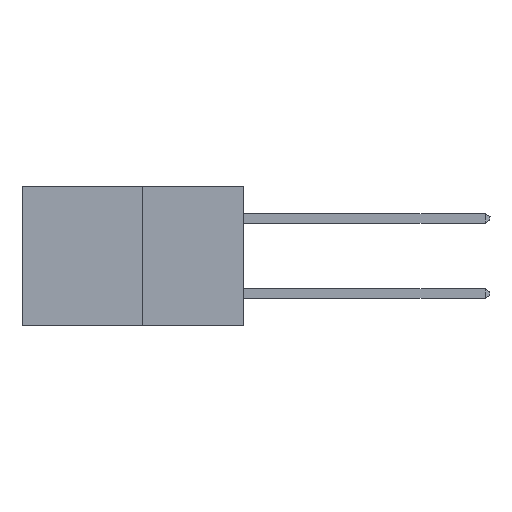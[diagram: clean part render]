
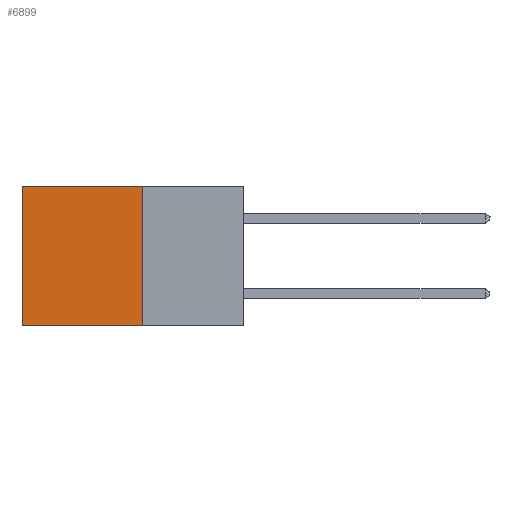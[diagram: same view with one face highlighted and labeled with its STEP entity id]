
A CAD part, left-side view. The second image highlights one B-rep face of the part: STEP entity #6899.
In plain terms, the highlighted planar face has unit normal (-1, 0, 0).
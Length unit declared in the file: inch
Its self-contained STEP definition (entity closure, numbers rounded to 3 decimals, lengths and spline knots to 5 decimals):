
#164 = LINE ( 'NONE', #6016, #4381 ) ;
#496 = VECTOR ( 'NONE', #9819, 39.37008 ) ;
#772 = LINE ( 'NONE', #3320, #496 ) ;
#805 = CARTESIAN_POINT ( 'NONE',  ( 0.277, 0.59, -0.37 ) ) ;
#1192 = DIRECTION ( 'NONE',  ( 0., 1., 0. ) ) ;
#1532 = CARTESIAN_POINT ( 'NONE',  ( 0.277, 0.27, -0.37 ) ) ;
#1769 = ORIENTED_EDGE ( 'NONE', *, *, #7540, .T. ) ;
#2384 = DIRECTION ( 'NONE',  ( 1., 0., 0. ) ) ;
#2575 = ORIENTED_EDGE ( 'NONE', *, *, #4249, .F. ) ;
#2632 = VERTEX_POINT ( 'NONE', #5399 ) ;
#3102 = VECTOR ( 'NONE', #1192, 39.37008 ) ;
#3320 = CARTESIAN_POINT ( 'NONE',  ( 0.277, 0.59, -0.37 ) ) ;
#3494 = EDGE_LOOP ( 'NONE', ( #1769, #8615, #2575, #4795 ) ) ;
#3533 = VERTEX_POINT ( 'NONE', #805 ) ;
#3874 = VERTEX_POINT ( 'NONE', #8811 ) ;
#3890 = LINE ( 'NONE', #7828, #3102 ) ;
#4249 = EDGE_CURVE ( 'NONE', #10524, #3874, #164, .T. ) ;
#4381 = VECTOR ( 'NONE', #6841, 39.37008 ) ;
#4795 = ORIENTED_EDGE ( 'NONE', *, *, #7093, .T. ) ;
#4980 = CARTESIAN_POINT ( 'NONE',  ( 0.277, 0.27, 0. ) ) ;
#5170 = DIRECTION ( 'NONE',  ( 0., 1., 0. ) ) ;
#5284 = AXIS2_PLACEMENT_3D ( 'NONE', #1532, #2384, #8138 ) ;
#5399 = CARTESIAN_POINT ( 'NONE',  ( 0.277, 0.59, 0. ) ) ;
#6016 = CARTESIAN_POINT ( 'NONE',  ( 0.277, 0.27, -0.37 ) ) ;
#6521 = PLANE ( 'NONE',  #5284 ) ;
#6645 = VECTOR ( 'NONE', #5170, 39.37008 ) ;
#6841 = DIRECTION ( 'NONE',  ( 0., 0., -1. ) ) ;
#6899 = ADVANCED_FACE ( 'NONE', ( #8672 ), #6521, .F. ) ;
#7093 = EDGE_CURVE ( 'NONE', #10524, #2632, #8793, .T. ) ;
#7540 = EDGE_CURVE ( 'NONE', #2632, #3533, #772, .T. ) ;
#7828 = CARTESIAN_POINT ( 'NONE',  ( 0.277, 0.27, -0.37 ) ) ;
#8138 = DIRECTION ( 'NONE',  ( 0., 0., -1. ) ) ;
#8415 = CARTESIAN_POINT ( 'NONE',  ( 0.277, 0.27, 0. ) ) ;
#8615 = ORIENTED_EDGE ( 'NONE', *, *, #10168, .F. ) ;
#8672 = FACE_OUTER_BOUND ( 'NONE', #3494, .T. ) ;
#8793 = LINE ( 'NONE', #8415, #6645 ) ;
#8811 = CARTESIAN_POINT ( 'NONE',  ( 0.277, 0.27, -0.37 ) ) ;
#9819 = DIRECTION ( 'NONE',  ( 0., 0., -1. ) ) ;
#10168 = EDGE_CURVE ( 'NONE', #3874, #3533, #3890, .T. ) ;
#10524 = VERTEX_POINT ( 'NONE', #4980 ) ;
